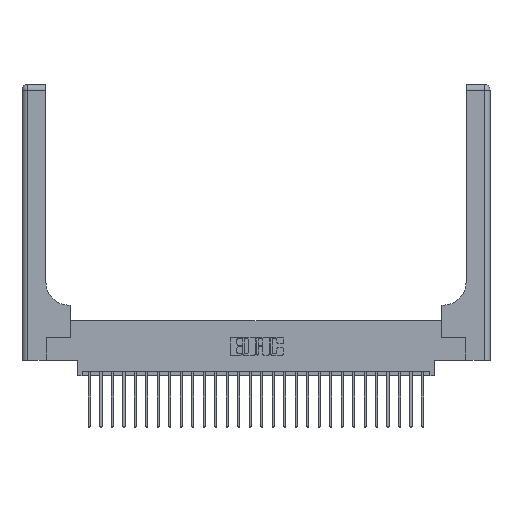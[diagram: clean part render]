
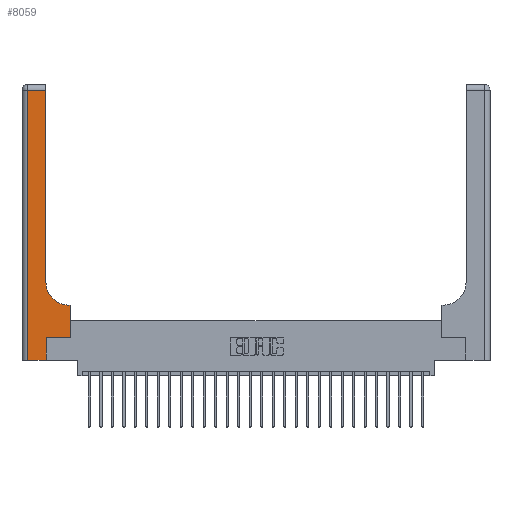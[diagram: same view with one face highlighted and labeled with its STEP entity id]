
A CAD part, top view. The second image highlights one B-rep face of the part: STEP entity #8059.
In plain terms, the highlighted planar face has unit normal (0, 0, 1).
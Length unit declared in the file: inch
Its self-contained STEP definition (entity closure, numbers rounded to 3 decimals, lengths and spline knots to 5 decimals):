
#507 = CARTESIAN_POINT ( 'NONE',  ( 0.06, 3., 0.37 ) ) ;
#520 = CARTESIAN_POINT ( 'NONE',  ( 0.26, 2.94, 0.37 ) ) ;
#594 = LINE ( 'NONE', #13039, #20835 ) ;
#631 = DIRECTION ( 'NONE',  ( 0., 0., -1. ) ) ;
#976 = CARTESIAN_POINT ( 'NONE',  ( 0.265, 0.25, 0.37 ) ) ;
#1095 = LINE ( 'NONE', #4560, #2096 ) ;
#1327 = EDGE_CURVE ( 'NONE', #8081, #23948, #21300, .T. ) ;
#1588 = CARTESIAN_POINT ( 'NONE',  ( 0.528, 0.25, 0.37 ) ) ;
#1718 = LINE ( 'NONE', #22744, #7861 ) ;
#2096 = VECTOR ( 'NONE', #17735, 39.37008 ) ;
#2300 = EDGE_CURVE ( 'NONE', #23948, #20892, #1718, .T. ) ;
#2376 = ORIENTED_EDGE ( 'NONE', *, *, #2992, .T. ) ;
#2992 = EDGE_CURVE ( 'NONE', #4502, #14020, #7278, .T. ) ;
#3167 = DIRECTION ( 'NONE',  ( -1., 0., 0. ) ) ;
#3780 = CARTESIAN_POINT ( 'NONE',  ( 0.26, 0.6, 0.37 ) ) ;
#3976 = CARTESIAN_POINT ( 'NONE',  ( 0.528, 0.6, 0.37 ) ) ;
#4412 = VERTEX_POINT ( 'NONE', #3976 ) ;
#4502 = VERTEX_POINT ( 'NONE', #6319 ) ;
#4560 = CARTESIAN_POINT ( 'NONE',  ( 0.265, 0., 0.37 ) ) ;
#5275 = CARTESIAN_POINT ( 'NONE',  ( 0., 3., 0.37 ) ) ;
#6220 = CARTESIAN_POINT ( 'NONE',  ( 0.265, 0., 0.37 ) ) ;
#6319 = CARTESIAN_POINT ( 'NONE',  ( 0.265, 0.25, 0.37 ) ) ;
#6549 = LINE ( 'NONE', #507, #23093 ) ;
#6764 = CARTESIAN_POINT ( 'NONE',  ( 0., 0., 0.37 ) ) ;
#7157 = EDGE_CURVE ( 'NONE', #10272, #4502, #1095, .T. ) ;
#7235 = EDGE_CURVE ( 'NONE', #20892, #18620, #594, .T. ) ;
#7278 = LINE ( 'NONE', #976, #13175 ) ;
#7328 = VERTEX_POINT ( 'NONE', #26881 ) ;
#7861 = VECTOR ( 'NONE', #18363, 39.37008 ) ;
#8059 = ADVANCED_FACE ( 'NONE', ( #13225 ), #23450, .F. ) ;
#8081 = VERTEX_POINT ( 'NONE', #11960 ) ;
#9315 = DIRECTION ( 'NONE',  ( 1., 0., 0. ) ) ;
#10272 = VERTEX_POINT ( 'NONE', #6220 ) ;
#10312 = CARTESIAN_POINT ( 'NONE',  ( 0.26, 0.85, 0.37 ) ) ;
#10484 = EDGE_CURVE ( 'NONE', #7328, #10272, #17499, .T. ) ;
#11534 = DIRECTION ( 'NONE',  ( 0., 0., -1. ) ) ;
#11602 = EDGE_LOOP ( 'NONE', ( #14318, #20336, #25890, #20744, #24388, #2376, #14522, #25112, #17748 ) ) ;
#11734 = LINE ( 'NONE', #17855, #15945 ) ;
#11741 = VECTOR ( 'NONE', #24802, 39.37008 ) ;
#11792 = VECTOR ( 'NONE', #19153, 39.37008 ) ;
#11960 = CARTESIAN_POINT ( 'NONE',  ( 0.51, 0.6, 0.37 ) ) ;
#13039 = CARTESIAN_POINT ( 'NONE',  ( 0., 2.94, 0.37 ) ) ;
#13175 = VECTOR ( 'NONE', #9315, 39.37008 ) ;
#13225 = FACE_OUTER_BOUND ( 'NONE', #11602, .T. ) ;
#13656 = DIRECTION ( 'NONE',  ( 0., 1., 0. ) ) ;
#14020 = VERTEX_POINT ( 'NONE', #1588 ) ;
#14318 = ORIENTED_EDGE ( 'NONE', *, *, #2300, .T. ) ;
#14522 = ORIENTED_EDGE ( 'NONE', *, *, #25519, .T. ) ;
#15008 = EDGE_CURVE ( 'NONE', #18620, #7328, #6549, .T. ) ;
#15287 = EDGE_CURVE ( 'NONE', #4412, #8081, #26567, .T. ) ;
#15945 = VECTOR ( 'NONE', #13656, 39.37008 ) ;
#17149 = DIRECTION ( 'NONE',  ( 0., -1., 0. ) ) ;
#17340 = AXIS2_PLACEMENT_3D ( 'NONE', #25888, #11534, #19834 ) ;
#17499 = LINE ( 'NONE', #6764, #11792 ) ;
#17735 = DIRECTION ( 'NONE',  ( 0., 1., 0. ) ) ;
#17748 = ORIENTED_EDGE ( 'NONE', *, *, #1327, .T. ) ;
#17855 = CARTESIAN_POINT ( 'NONE',  ( 0.528, 0.25, 0.37 ) ) ;
#18363 = DIRECTION ( 'NONE',  ( 0., 1., 0. ) ) ;
#18620 = VERTEX_POINT ( 'NONE', #19983 ) ;
#19153 = DIRECTION ( 'NONE',  ( 1., 0., 0. ) ) ;
#19834 = DIRECTION ( 'NONE',  ( 1., 0., 0. ) ) ;
#19983 = CARTESIAN_POINT ( 'NONE',  ( 0.06, 2.94, 0.37 ) ) ;
#20336 = ORIENTED_EDGE ( 'NONE', *, *, #7235, .T. ) ;
#20744 = ORIENTED_EDGE ( 'NONE', *, *, #10484, .T. ) ;
#20835 = VECTOR ( 'NONE', #3167, 39.37008 ) ;
#20892 = VERTEX_POINT ( 'NONE', #520 ) ;
#21300 = CIRCLE ( 'NONE', #17340, 0.25 ) ;
#22744 = CARTESIAN_POINT ( 'NONE',  ( 0.26, 3., 0.37 ) ) ;
#23093 = VECTOR ( 'NONE', #17149, 39.37008 ) ;
#23450 = PLANE ( 'NONE',  #25596 ) ;
#23948 = VERTEX_POINT ( 'NONE', #10312 ) ;
#24388 = ORIENTED_EDGE ( 'NONE', *, *, #7157, .T. ) ;
#24802 = DIRECTION ( 'NONE',  ( -1., 0., 0. ) ) ;
#25112 = ORIENTED_EDGE ( 'NONE', *, *, #15287, .T. ) ;
#25519 = EDGE_CURVE ( 'NONE', #14020, #4412, #11734, .T. ) ;
#25596 = AXIS2_PLACEMENT_3D ( 'NONE', #5275, #631, #25638 ) ;
#25638 = DIRECTION ( 'NONE',  ( -1., 0., 0. ) ) ;
#25888 = CARTESIAN_POINT ( 'NONE',  ( 0.51, 0.85, 0.37 ) ) ;
#25890 = ORIENTED_EDGE ( 'NONE', *, *, #15008, .T. ) ;
#26567 = LINE ( 'NONE', #3780, #11741 ) ;
#26881 = CARTESIAN_POINT ( 'NONE',  ( 0.06, 0., 0.37 ) ) ;
